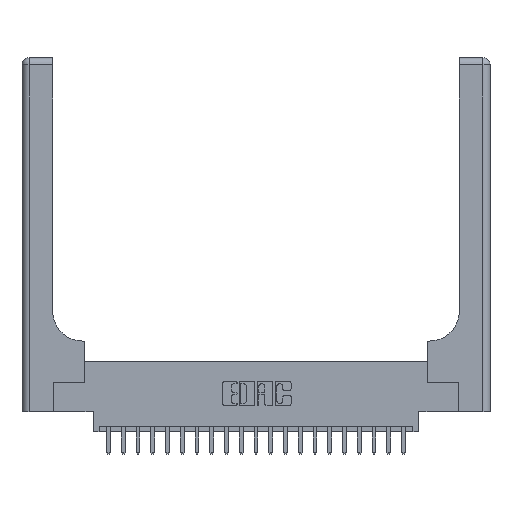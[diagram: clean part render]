
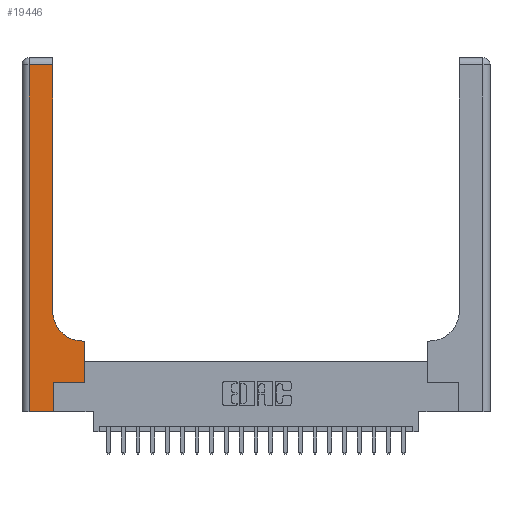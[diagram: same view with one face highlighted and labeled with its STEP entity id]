
A CAD part, top view. The second image highlights one B-rep face of the part: STEP entity #19446.
In plain terms, the highlighted planar face has unit normal (0, 0, 1).
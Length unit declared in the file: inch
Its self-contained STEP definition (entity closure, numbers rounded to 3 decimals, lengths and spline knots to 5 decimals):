
#205 = DIRECTION ( 'NONE',  ( -1., 0., 0. ) ) ;
#325 = EDGE_CURVE ( 'NONE', #4043, #15167, #20944, .T. ) ;
#437 = DIRECTION ( 'NONE',  ( 1., 0., 0. ) ) ;
#925 = CARTESIAN_POINT ( 'NONE',  ( 0.265, 0., 0.37 ) ) ;
#1441 = VECTOR ( 'NONE', #16511, 39.37008 ) ;
#2345 = LINE ( 'NONE', #10704, #15631 ) ;
#2408 = VECTOR ( 'NONE', #13251, 39.37008 ) ;
#2725 = CARTESIAN_POINT ( 'NONE',  ( 0.26, 3., 0.37 ) ) ;
#2744 = VERTEX_POINT ( 'NONE', #11814 ) ;
#2958 = CARTESIAN_POINT ( 'NONE',  ( 0.26, 0.85, 0.37 ) ) ;
#3009 = VECTOR ( 'NONE', #4706, 39.37008 ) ;
#3186 = CARTESIAN_POINT ( 'NONE',  ( 0., 0., 0.37 ) ) ;
#3433 = VECTOR ( 'NONE', #6271, 39.37008 ) ;
#3811 = ORIENTED_EDGE ( 'NONE', *, *, #18257, .T. ) ;
#3992 = EDGE_CURVE ( 'NONE', #2744, #8704, #14381, .T. ) ;
#4043 = VERTEX_POINT ( 'NONE', #17699 ) ;
#4413 = AXIS2_PLACEMENT_3D ( 'NONE', #20859, #10933, #437 ) ;
#4706 = DIRECTION ( 'NONE',  ( -1., 0., 0. ) ) ;
#5105 = DIRECTION ( 'NONE',  ( -1., 0., 0. ) ) ;
#6178 = FACE_OUTER_BOUND ( 'NONE', #19098, .T. ) ;
#6271 = DIRECTION ( 'NONE',  ( 0., 1., 0. ) ) ;
#6950 = CARTESIAN_POINT ( 'NONE',  ( 0.06, 3., 0.37 ) ) ;
#7115 = ORIENTED_EDGE ( 'NONE', *, *, #15841, .T. ) ;
#7569 = VECTOR ( 'NONE', #12004, 39.37008 ) ;
#7705 = LINE ( 'NONE', #8238, #3009 ) ;
#8127 = LINE ( 'NONE', #925, #3433 ) ;
#8238 = CARTESIAN_POINT ( 'NONE',  ( 0., 2.94, 0.37 ) ) ;
#8568 = ORIENTED_EDGE ( 'NONE', *, *, #19971, .T. ) ;
#8704 = VERTEX_POINT ( 'NONE', #2958 ) ;
#8724 = ORIENTED_EDGE ( 'NONE', *, *, #325, .T. ) ;
#8967 = CARTESIAN_POINT ( 'NONE',  ( 0.06, 0., 0.37 ) ) ;
#9331 = LINE ( 'NONE', #3186, #7569 ) ;
#9495 = LINE ( 'NONE', #6950, #11103 ) ;
#10133 = EDGE_CURVE ( 'NONE', #20328, #13213, #9331, .T. ) ;
#10704 = CARTESIAN_POINT ( 'NONE',  ( 0.26, 0.6, 0.37 ) ) ;
#10752 = DIRECTION ( 'NONE',  ( 1., 0., 0. ) ) ;
#10808 = CARTESIAN_POINT ( 'NONE',  ( 0.265, 0.25, 0.37 ) ) ;
#10933 = DIRECTION ( 'NONE',  ( 0., 0., -1. ) ) ;
#11063 = VERTEX_POINT ( 'NONE', #21043 ) ;
#11103 = VECTOR ( 'NONE', #13831, 39.37008 ) ;
#11522 = CARTESIAN_POINT ( 'NONE',  ( 0.528, 0.25, 0.37 ) ) ;
#11674 = ORIENTED_EDGE ( 'NONE', *, *, #18822, .T. ) ;
#11814 = CARTESIAN_POINT ( 'NONE',  ( 0.51, 0.6, 0.37 ) ) ;
#12004 = DIRECTION ( 'NONE',  ( 1., 0., 0. ) ) ;
#12005 = ORIENTED_EDGE ( 'NONE', *, *, #3992, .T. ) ;
#12123 = EDGE_CURVE ( 'NONE', #13213, #4043, #8127, .T. ) ;
#12344 = ORIENTED_EDGE ( 'NONE', *, *, #10133, .T. ) ;
#13121 = ORIENTED_EDGE ( 'NONE', *, *, #16808, .T. ) ;
#13213 = VERTEX_POINT ( 'NONE', #15810 ) ;
#13251 = DIRECTION ( 'NONE',  ( 0., 1., 0. ) ) ;
#13831 = DIRECTION ( 'NONE',  ( 0., -1., 0. ) ) ;
#14381 = CIRCLE ( 'NONE', #4413, 0.25 ) ;
#14532 = CARTESIAN_POINT ( 'NONE',  ( 0.528, 0.6, 0.37 ) ) ;
#14931 = CARTESIAN_POINT ( 'NONE',  ( 0.06, 2.94, 0.37 ) ) ;
#15010 = CARTESIAN_POINT ( 'NONE',  ( 0.528, 0.25, 0.37 ) ) ;
#15167 = VERTEX_POINT ( 'NONE', #15010 ) ;
#15411 = DIRECTION ( 'NONE',  ( 0., 0., -1. ) ) ;
#15631 = VECTOR ( 'NONE', #205, 39.37008 ) ;
#15810 = CARTESIAN_POINT ( 'NONE',  ( 0.265, 0., 0.37 ) ) ;
#15841 = EDGE_CURVE ( 'NONE', #11063, #17355, #7705, .T. ) ;
#16186 = LINE ( 'NONE', #11522, #2408 ) ;
#16511 = DIRECTION ( 'NONE',  ( 0., 1., 0. ) ) ;
#16602 = VECTOR ( 'NONE', #10752, 39.37008 ) ;
#16808 = EDGE_CURVE ( 'NONE', #15167, #21910, #16186, .T. ) ;
#16867 = ORIENTED_EDGE ( 'NONE', *, *, #12123, .T. ) ;
#17355 = VERTEX_POINT ( 'NONE', #14931 ) ;
#17384 = AXIS2_PLACEMENT_3D ( 'NONE', #20183, #15411, #5105 ) ;
#17699 = CARTESIAN_POINT ( 'NONE',  ( 0.265, 0.25, 0.37 ) ) ;
#18257 = EDGE_CURVE ( 'NONE', #21910, #2744, #2345, .T. ) ;
#18822 = EDGE_CURVE ( 'NONE', #17355, #20328, #9495, .T. ) ;
#19098 = EDGE_LOOP ( 'NONE', ( #8568, #7115, #11674, #12344, #16867, #8724, #13121, #3811, #12005 ) ) ;
#19111 = LINE ( 'NONE', #2725, #1441 ) ;
#19446 = ADVANCED_FACE ( 'NONE', ( #6178 ), #21840, .F. ) ;
#19971 = EDGE_CURVE ( 'NONE', #8704, #11063, #19111, .T. ) ;
#20183 = CARTESIAN_POINT ( 'NONE',  ( 0., 3., 0.37 ) ) ;
#20328 = VERTEX_POINT ( 'NONE', #8967 ) ;
#20859 = CARTESIAN_POINT ( 'NONE',  ( 0.51, 0.85, 0.37 ) ) ;
#20944 = LINE ( 'NONE', #10808, #16602 ) ;
#21043 = CARTESIAN_POINT ( 'NONE',  ( 0.26, 2.94, 0.37 ) ) ;
#21840 = PLANE ( 'NONE',  #17384 ) ;
#21910 = VERTEX_POINT ( 'NONE', #14532 ) ;
